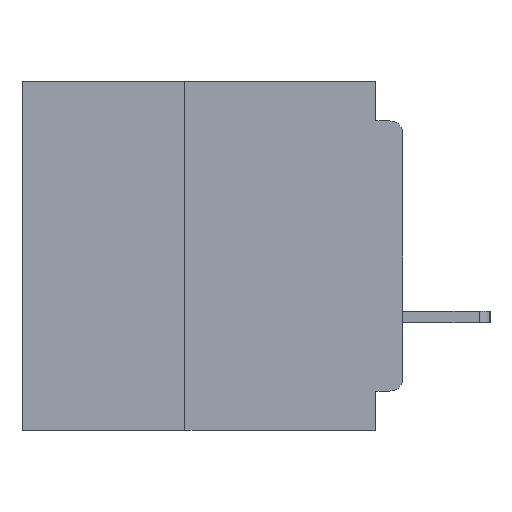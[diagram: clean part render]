
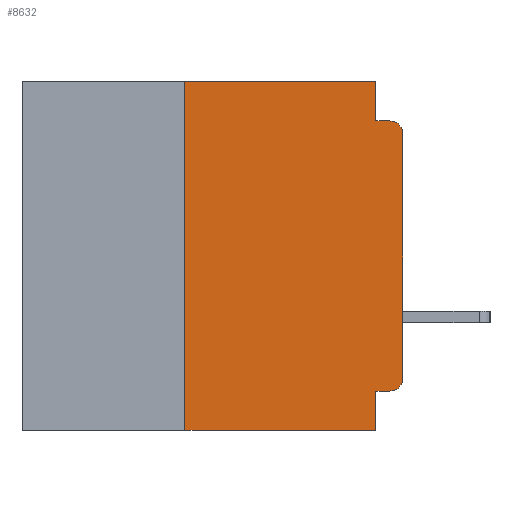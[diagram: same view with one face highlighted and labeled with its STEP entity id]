
A CAD part, left-side view. The second image highlights one B-rep face of the part: STEP entity #8632.
In plain terms, the highlighted planar face has unit normal (-1, 0, 0).
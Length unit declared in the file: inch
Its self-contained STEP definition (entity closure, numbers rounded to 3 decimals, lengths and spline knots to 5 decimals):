
#209 = EDGE_LOOP ( 'NONE', ( #24501, #24463, #32097, #3127, #29457, #34042, #29342, #21577, #25581, #13116 ) ) ;
#299 = EDGE_CURVE ( 'NONE', #17289, #25157, #24687, .T. ) ;
#411 = LINE ( 'NONE', #33883, #6128 ) ;
#1354 = DIRECTION ( 'NONE',  ( -1., 0., 0. ) ) ;
#1822 = VERTEX_POINT ( 'NONE', #20098 ) ;
#2852 = DIRECTION ( 'NONE',  ( 0., 0., 1. ) ) ;
#3127 = ORIENTED_EDGE ( 'NONE', *, *, #16568, .F. ) ;
#3173 = CARTESIAN_POINT ( 'NONE',  ( 0., 0.031, 0. ) ) ;
#3834 = CARTESIAN_POINT ( 'NONE',  ( 0., 0.25, 0. ) ) ;
#4960 = VECTOR ( 'NONE', #7497, 39.37008 ) ;
#6128 = VECTOR ( 'NONE', #20230, 39.37008 ) ;
#6290 = CARTESIAN_POINT ( 'NONE',  ( 0., 0.031, -0.355 ) ) ;
#6501 = VERTEX_POINT ( 'NONE', #6290 ) ;
#6589 = VERTEX_POINT ( 'NONE', #3834 ) ;
#6874 = CARTESIAN_POINT ( 'NONE',  ( 0., 0.437, 0. ) ) ;
#7194 = FACE_OUTER_BOUND ( 'NONE', #209, .T. ) ;
#7497 = DIRECTION ( 'NONE',  ( 0., 1., 0. ) ) ;
#7566 = CARTESIAN_POINT ( 'NONE',  ( 0., 0., -0.06 ) ) ;
#7652 = CARTESIAN_POINT ( 'NONE',  ( 0., 0.015, -0.045 ) ) ;
#8632 = ADVANCED_FACE ( 'NONE', ( #7194 ), #23530, .F. ) ;
#8633 = EDGE_CURVE ( 'NONE', #27629, #14900, #29325, .T. ) ;
#9500 = DIRECTION ( 'NONE',  ( 1., 0., 0. ) ) ;
#9629 = DIRECTION ( 'NONE',  ( 0., 0., -1. ) ) ;
#9892 = LINE ( 'NONE', #3173, #31126 ) ;
#11396 = DIRECTION ( 'NONE',  ( 0., 0., -1. ) ) ;
#11481 = EDGE_CURVE ( 'NONE', #6589, #18147, #20771, .T. ) ;
#11584 = EDGE_CURVE ( 'NONE', #6501, #25157, #31914, .T. ) ;
#12223 = VERTEX_POINT ( 'NONE', #35296 ) ;
#12433 = DIRECTION ( 'NONE',  ( 0., -1., 0. ) ) ;
#12718 = CARTESIAN_POINT ( 'NONE',  ( 0., 0.437, -0.4 ) ) ;
#13075 = CARTESIAN_POINT ( 'NONE',  ( 0., 0.437, 0. ) ) ;
#13116 = ORIENTED_EDGE ( 'NONE', *, *, #14276, .T. ) ;
#13396 = VECTOR ( 'NONE', #32369, 39.37008 ) ;
#13687 = EDGE_CURVE ( 'NONE', #1822, #6501, #19719, .T. ) ;
#14276 = EDGE_CURVE ( 'NONE', #1822, #29122, #27462, .T. ) ;
#14529 = CARTESIAN_POINT ( 'NONE',  ( 0., 0., -0.045 ) ) ;
#14900 = VERTEX_POINT ( 'NONE', #7652 ) ;
#15973 = CARTESIAN_POINT ( 'NONE',  ( 0., 0.015, -0.34 ) ) ;
#16568 = EDGE_CURVE ( 'NONE', #18147, #12223, #9892, .T. ) ;
#17289 = VERTEX_POINT ( 'NONE', #23160 ) ;
#18053 = CARTESIAN_POINT ( 'NONE',  ( 0., 0.015, -0.06 ) ) ;
#18147 = VERTEX_POINT ( 'NONE', #27556 ) ;
#18762 = DIRECTION ( 'NONE',  ( 0., 0., -1. ) ) ;
#19719 = LINE ( 'NONE', #26927, #4960 ) ;
#20098 = CARTESIAN_POINT ( 'NONE',  ( 0., 0.015, -0.355 ) ) ;
#20230 = DIRECTION ( 'NONE',  ( 0., 0., 1. ) ) ;
#20771 = LINE ( 'NONE', #13075, #13396 ) ;
#20833 = DIRECTION ( 'NONE',  ( 0., 0., -1. ) ) ;
#21577 = ORIENTED_EDGE ( 'NONE', *, *, #11584, .F. ) ;
#21808 = DIRECTION ( 'NONE',  ( 0., 0., -1. ) ) ;
#21955 = AXIS2_PLACEMENT_3D ( 'NONE', #15973, #35187, #18762 ) ;
#22429 = CARTESIAN_POINT ( 'NONE',  ( 0., 0., -0.34 ) ) ;
#23160 = CARTESIAN_POINT ( 'NONE',  ( 0., 0.25, -0.4 ) ) ;
#23198 = LINE ( 'NONE', #14529, #31333 ) ;
#23530 = PLANE ( 'NONE',  #28305 ) ;
#24463 = ORIENTED_EDGE ( 'NONE', *, *, #8633, .T. ) ;
#24501 = ORIENTED_EDGE ( 'NONE', *, *, #26598, .T. ) ;
#24687 = LINE ( 'NONE', #12718, #31909 ) ;
#25157 = VERTEX_POINT ( 'NONE', #27589 ) ;
#25581 = ORIENTED_EDGE ( 'NONE', *, *, #13687, .F. ) ;
#26466 = AXIS2_PLACEMENT_3D ( 'NONE', #18053, #1354, #20833 ) ;
#26598 = EDGE_CURVE ( 'NONE', #29122, #27629, #411, .T. ) ;
#26616 = VECTOR ( 'NONE', #2852, 39.37008 ) ;
#26927 = CARTESIAN_POINT ( 'NONE',  ( 0., 0., -0.355 ) ) ;
#27387 = CARTESIAN_POINT ( 'NONE',  ( 0., 0.031, -0.4 ) ) ;
#27462 = CIRCLE ( 'NONE', #21955, 0.015 ) ;
#27556 = CARTESIAN_POINT ( 'NONE',  ( 0., 0.031, 0. ) ) ;
#27589 = CARTESIAN_POINT ( 'NONE',  ( 0., 0.031, -0.4 ) ) ;
#27629 = VERTEX_POINT ( 'NONE', #7566 ) ;
#28305 = AXIS2_PLACEMENT_3D ( 'NONE', #6874, #9500, #9629 ) ;
#29122 = VERTEX_POINT ( 'NONE', #22429 ) ;
#29177 = EDGE_CURVE ( 'NONE', #12223, #14900, #23198, .T. ) ;
#29325 = CIRCLE ( 'NONE', #26466, 0.015 ) ;
#29342 = ORIENTED_EDGE ( 'NONE', *, *, #299, .T. ) ;
#29457 = ORIENTED_EDGE ( 'NONE', *, *, #11481, .F. ) ;
#29586 = EDGE_CURVE ( 'NONE', #17289, #6589, #32987, .T. ) ;
#31126 = VECTOR ( 'NONE', #11396, 39.37008 ) ;
#31333 = VECTOR ( 'NONE', #33749, 39.37008 ) ;
#31909 = VECTOR ( 'NONE', #12433, 39.37008 ) ;
#31914 = LINE ( 'NONE', #27387, #33627 ) ;
#32097 = ORIENTED_EDGE ( 'NONE', *, *, #29177, .F. ) ;
#32369 = DIRECTION ( 'NONE',  ( 0., -1., 0. ) ) ;
#32987 = LINE ( 'NONE', #35891, #26616 ) ;
#33627 = VECTOR ( 'NONE', #21808, 39.37008 ) ;
#33749 = DIRECTION ( 'NONE',  ( 0., -1., 0. ) ) ;
#33883 = CARTESIAN_POINT ( 'NONE',  ( 0., 0., 0. ) ) ;
#34042 = ORIENTED_EDGE ( 'NONE', *, *, #29586, .F. ) ;
#35187 = DIRECTION ( 'NONE',  ( -1., 0., 0. ) ) ;
#35296 = CARTESIAN_POINT ( 'NONE',  ( 0., 0.031, -0.045 ) ) ;
#35891 = CARTESIAN_POINT ( 'NONE',  ( 0., 0.25, -0.4 ) ) ;
